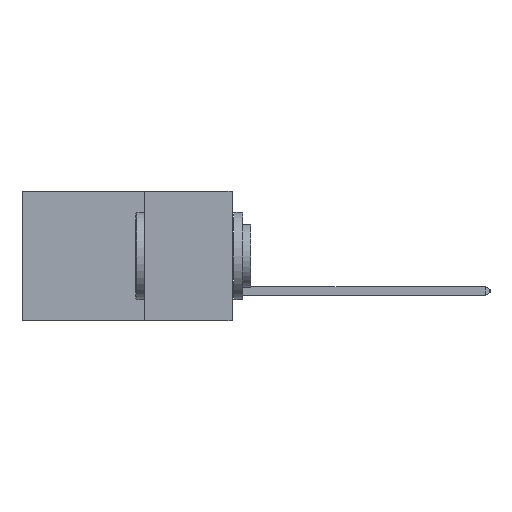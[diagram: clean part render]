
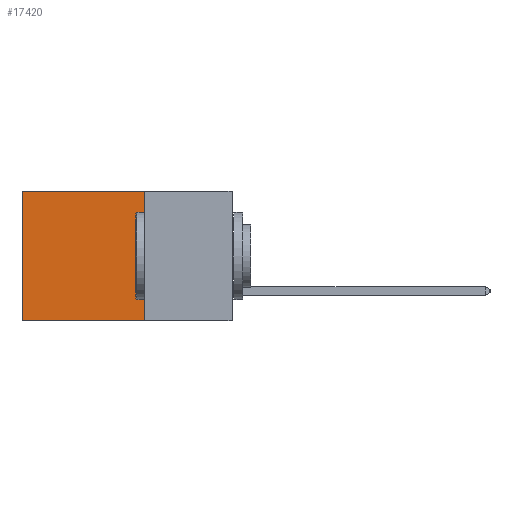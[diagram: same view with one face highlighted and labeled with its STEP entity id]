
A CAD part, left-side view. The second image highlights one B-rep face of the part: STEP entity #17420.
In plain terms, the highlighted planar face has unit normal (-1, 0, 0).
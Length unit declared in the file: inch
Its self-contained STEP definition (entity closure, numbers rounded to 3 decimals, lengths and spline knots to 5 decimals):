
#401 = DIRECTION ( 'NONE',  ( 0., 0., -1. ) ) ;
#1514 = ORIENTED_EDGE ( 'NONE', *, *, #26752, .F. ) ;
#1901 = CARTESIAN_POINT ( 'NONE',  ( 0.2875, 0.25, -0.37 ) ) ;
#2807 = DIRECTION ( 'NONE',  ( 1., 0., 0. ) ) ;
#3333 = DIRECTION ( 'NONE',  ( 0., 1., 0. ) ) ;
#3401 = VERTEX_POINT ( 'NONE', #14955 ) ;
#5016 = AXIS2_PLACEMENT_3D ( 'NONE', #27617, #2807, #22190 ) ;
#5730 = VECTOR ( 'NONE', #401, 39.37008 ) ;
#6261 = VECTOR ( 'NONE', #8065, 39.37008 ) ;
#7547 = VECTOR ( 'NONE', #3333, 39.37008 ) ;
#8065 = DIRECTION ( 'NONE',  ( 0., 1., 0. ) ) ;
#9169 = CARTESIAN_POINT ( 'NONE',  ( 0.2875, 0.6, 0. ) ) ;
#9454 = CARTESIAN_POINT ( 'NONE',  ( 0.2875, 0.25, 0. ) ) ;
#10765 = EDGE_CURVE ( 'NONE', #11485, #3401, #21348, .T. ) ;
#11485 = VERTEX_POINT ( 'NONE', #9169 ) ;
#13421 = LINE ( 'NONE', #9454, #33661 ) ;
#14668 = VERTEX_POINT ( 'NONE', #1901 ) ;
#14955 = CARTESIAN_POINT ( 'NONE',  ( 0.2875, 0.6, -0.37 ) ) ;
#15097 = VERTEX_POINT ( 'NONE', #31322 ) ;
#17248 = ORIENTED_EDGE ( 'NONE', *, *, #26556, .T. ) ;
#17420 = ADVANCED_FACE ( 'NONE', ( #21621 ), #19439, .F. ) ;
#18921 = ORIENTED_EDGE ( 'NONE', *, *, #10765, .T. ) ;
#19132 = ORIENTED_EDGE ( 'NONE', *, *, #23203, .F. ) ;
#19439 = PLANE ( 'NONE',  #5016 ) ;
#20155 = LINE ( 'NONE', #35579, #6261 ) ;
#21348 = LINE ( 'NONE', #22561, #5730 ) ;
#21621 = FACE_OUTER_BOUND ( 'NONE', #33107, .T. ) ;
#22190 = DIRECTION ( 'NONE',  ( 0., 0., -1. ) ) ;
#22561 = CARTESIAN_POINT ( 'NONE',  ( 0.2875, 0.6, 0. ) ) ;
#23203 = EDGE_CURVE ( 'NONE', #15097, #14668, #13421, .T. ) ;
#23370 = DIRECTION ( 'NONE',  ( 0., 0., -1. ) ) ;
#25490 = CARTESIAN_POINT ( 'NONE',  ( 0.2875, 0.25, -0.37 ) ) ;
#26556 = EDGE_CURVE ( 'NONE', #15097, #11485, #20155, .T. ) ;
#26752 = EDGE_CURVE ( 'NONE', #14668, #3401, #29605, .T. ) ;
#27617 = CARTESIAN_POINT ( 'NONE',  ( 0.2875, 0.25, 0. ) ) ;
#29605 = LINE ( 'NONE', #25490, #7547 ) ;
#31322 = CARTESIAN_POINT ( 'NONE',  ( 0.2875, 0.25, 0. ) ) ;
#33107 = EDGE_LOOP ( 'NONE', ( #18921, #1514, #19132, #17248 ) ) ;
#33661 = VECTOR ( 'NONE', #23370, 39.37008 ) ;
#35579 = CARTESIAN_POINT ( 'NONE',  ( 0.2875, 0.25, 0. ) ) ;
